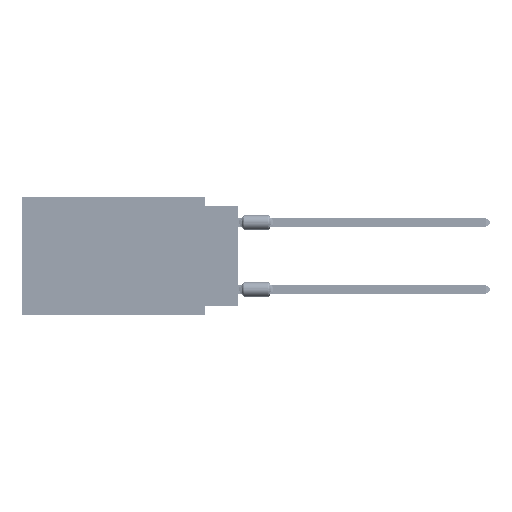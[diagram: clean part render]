
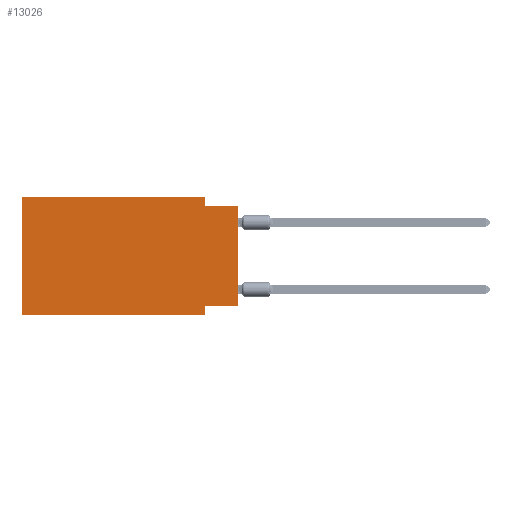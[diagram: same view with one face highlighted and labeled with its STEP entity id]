
A CAD part, left-side view. The second image highlights one B-rep face of the part: STEP entity #13026.
In plain terms, the highlighted planar face has unit normal (-1, 0, 0).
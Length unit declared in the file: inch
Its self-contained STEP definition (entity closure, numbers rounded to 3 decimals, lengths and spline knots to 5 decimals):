
#456 = ORIENTED_EDGE ( 'NONE', *, *, #60945, .F. ) ;
#2147 = VERTEX_POINT ( 'NONE', #50932 ) ;
#2375 = FACE_OUTER_BOUND ( 'NONE', #20492, .T. ) ;
#2974 = LINE ( 'NONE', #23604, #25341 ) ;
#5559 = VERTEX_POINT ( 'NONE', #24678 ) ;
#5590 = VECTOR ( 'NONE', #16925, 39.37008 ) ;
#9224 = LINE ( 'NONE', #51241, #37345 ) ;
#10997 = CARTESIAN_POINT ( 'NONE',  ( 0., 0.1, -0.325 ) ) ;
#11577 = CARTESIAN_POINT ( 'NONE',  ( 0., 0.1, -0.025 ) ) ;
#12148 = ORIENTED_EDGE ( 'NONE', *, *, #71307, .F. ) ;
#13026 = ADVANCED_FACE ( 'NONE', ( #2375 ), #56463, .F. ) ;
#14772 = LINE ( 'NONE', #26023, #69885 ) ;
#16170 = ORIENTED_EDGE ( 'NONE', *, *, #21549, .F. ) ;
#16925 = DIRECTION ( 'NONE',  ( 0., -1., 0. ) ) ;
#17185 = CARTESIAN_POINT ( 'NONE',  ( 0., 0.1, 0. ) ) ;
#17569 = CARTESIAN_POINT ( 'NONE',  ( 0., 0.645, -0.35 ) ) ;
#17823 = CARTESIAN_POINT ( 'NONE',  ( 0., 0., -0.325 ) ) ;
#19454 = DIRECTION ( 'NONE',  ( 0., 0., -1. ) ) ;
#20492 = EDGE_LOOP ( 'NONE', ( #44816, #70152, #39436, #16170, #12148, #57475, #456, #72072 ) ) ;
#20688 = DIRECTION ( 'NONE',  ( 0., 0., -1. ) ) ;
#21549 = EDGE_CURVE ( 'NONE', #5559, #69293, #14772, .T. ) ;
#21597 = LINE ( 'NONE', #38305, #71947 ) ;
#23520 = LINE ( 'NONE', #28197, #5590 ) ;
#23604 = CARTESIAN_POINT ( 'NONE',  ( 0., 0.645, 0. ) ) ;
#24678 = CARTESIAN_POINT ( 'NONE',  ( 0., 0.645, 0. ) ) ;
#24994 = EDGE_CURVE ( 'NONE', #74225, #45879, #47742, .T. ) ;
#25341 = VECTOR ( 'NONE', #34880, 39.37008 ) ;
#26023 = CARTESIAN_POINT ( 'NONE',  ( 0., 0.645, 0. ) ) ;
#28197 = CARTESIAN_POINT ( 'NONE',  ( 0., 0., -0.025 ) ) ;
#28199 = AXIS2_PLACEMENT_3D ( 'NONE', #33131, #73966, #20688 ) ;
#29000 = LINE ( 'NONE', #52729, #65375 ) ;
#29757 = DIRECTION ( 'NONE',  ( 0., -1., 0. ) ) ;
#33131 = CARTESIAN_POINT ( 'NONE',  ( 0., 0.645, 0. ) ) ;
#34880 = DIRECTION ( 'NONE',  ( 0., 0., 1. ) ) ;
#34897 = CARTESIAN_POINT ( 'NONE',  ( 0., 0.1, -0.35 ) ) ;
#36331 = CARTESIAN_POINT ( 'NONE',  ( 0., 0., -0.325 ) ) ;
#37345 = VECTOR ( 'NONE', #56274, 39.37008 ) ;
#38305 = CARTESIAN_POINT ( 'NONE',  ( 0., 0.1, 0. ) ) ;
#39436 = ORIENTED_EDGE ( 'NONE', *, *, #65792, .F. ) ;
#43157 = DIRECTION ( 'NONE',  ( 0., -1., 0. ) ) ;
#44816 = ORIENTED_EDGE ( 'NONE', *, *, #53364, .T. ) ;
#45879 = VERTEX_POINT ( 'NONE', #10997 ) ;
#47742 = LINE ( 'NONE', #17823, #52641 ) ;
#49383 = LINE ( 'NONE', #60304, #66497 ) ;
#50932 = CARTESIAN_POINT ( 'NONE',  ( 0., 0., -0.025 ) ) ;
#51241 = CARTESIAN_POINT ( 'NONE',  ( 0., 0., 0. ) ) ;
#51553 = DIRECTION ( 'NONE',  ( 0., 0., -1. ) ) ;
#52641 = VECTOR ( 'NONE', #59790, 39.37008 ) ;
#52729 = CARTESIAN_POINT ( 'NONE',  ( 0., 0.645, -0.35 ) ) ;
#53364 = EDGE_CURVE ( 'NONE', #74225, #2147, #9224, .T. ) ;
#54812 = VERTEX_POINT ( 'NONE', #34897 ) ;
#56274 = DIRECTION ( 'NONE',  ( 0., 0., 1. ) ) ;
#56463 = PLANE ( 'NONE',  #28199 ) ;
#57475 = ORIENTED_EDGE ( 'NONE', *, *, #75377, .T. ) ;
#58292 = VERTEX_POINT ( 'NONE', #11577 ) ;
#58675 = EDGE_CURVE ( 'NONE', #58292, #2147, #23520, .T. ) ;
#59790 = DIRECTION ( 'NONE',  ( 0., 1., 0. ) ) ;
#60304 = CARTESIAN_POINT ( 'NONE',  ( 0., 0.1, -0.35 ) ) ;
#60945 = EDGE_CURVE ( 'NONE', #45879, #54812, #49383, .T. ) ;
#65375 = VECTOR ( 'NONE', #29757, 39.37008 ) ;
#65792 = EDGE_CURVE ( 'NONE', #69293, #58292, #21597, .T. ) ;
#66497 = VECTOR ( 'NONE', #19454, 39.37008 ) ;
#69232 = VERTEX_POINT ( 'NONE', #17569 ) ;
#69293 = VERTEX_POINT ( 'NONE', #17185 ) ;
#69885 = VECTOR ( 'NONE', #43157, 39.37008 ) ;
#70152 = ORIENTED_EDGE ( 'NONE', *, *, #58675, .F. ) ;
#71307 = EDGE_CURVE ( 'NONE', #69232, #5559, #2974, .T. ) ;
#71947 = VECTOR ( 'NONE', #51553, 39.37008 ) ;
#72072 = ORIENTED_EDGE ( 'NONE', *, *, #24994, .F. ) ;
#73966 = DIRECTION ( 'NONE',  ( 1., 0., 0. ) ) ;
#74225 = VERTEX_POINT ( 'NONE', #36331 ) ;
#75377 = EDGE_CURVE ( 'NONE', #69232, #54812, #29000, .T. ) ;
